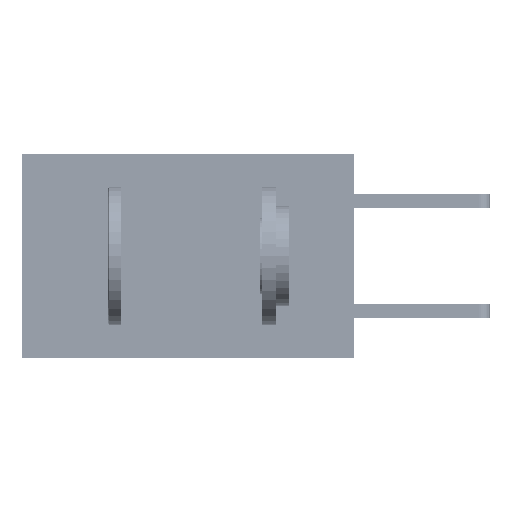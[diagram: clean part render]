
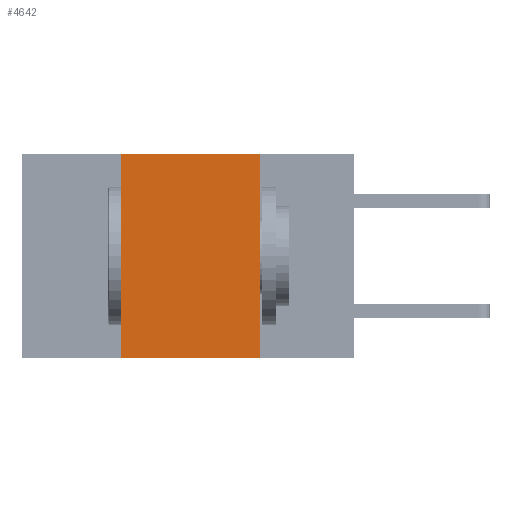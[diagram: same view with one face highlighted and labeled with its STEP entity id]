
A CAD part, left-side view. The second image highlights one B-rep face of the part: STEP entity #4642.
In plain terms, the highlighted planar face has unit normal (-1, 0, 0).
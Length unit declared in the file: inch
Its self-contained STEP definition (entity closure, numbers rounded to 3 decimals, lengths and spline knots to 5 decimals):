
#1347 = VERTEX_POINT ( 'NONE', #31128 ) ;
#1483 = CARTESIAN_POINT ( 'NONE',  ( 0., 0.17, 0. ) ) ;
#2092 = DIRECTION ( 'NONE',  ( 1., 0., 0. ) ) ;
#2954 = LINE ( 'NONE', #18787, #37682 ) ;
#4218 = DIRECTION ( 'NONE',  ( 0., -1., 0. ) ) ;
#4642 = ADVANCED_FACE ( 'NONE', ( #6497 ), #38147, .F. ) ;
#6009 = ORIENTED_EDGE ( 'NONE', *, *, #40248, .F. ) ;
#6497 = FACE_OUTER_BOUND ( 'NONE', #8638, .T. ) ;
#8426 = VERTEX_POINT ( 'NONE', #46338 ) ;
#8638 = EDGE_LOOP ( 'NONE', ( #23940, #8765, #6009, #19780 ) ) ;
#8765 = ORIENTED_EDGE ( 'NONE', *, *, #28833, .F. ) ;
#12913 = LINE ( 'NONE', #1483, #31798 ) ;
#18787 = CARTESIAN_POINT ( 'NONE',  ( 0., 0.6, 0. ) ) ;
#19563 = DIRECTION ( 'NONE',  ( 0., -1., 0. ) ) ;
#19780 = ORIENTED_EDGE ( 'NONE', *, *, #46282, .T. ) ;
#19797 = LINE ( 'NONE', #47793, #23349 ) ;
#20001 = CARTESIAN_POINT ( 'NONE',  ( 0., 0.42, 0. ) ) ;
#20131 = CARTESIAN_POINT ( 'NONE',  ( 0., 0.42, -0.37 ) ) ;
#23349 = VECTOR ( 'NONE', #4218, 39.37008 ) ;
#23940 = ORIENTED_EDGE ( 'NONE', *, *, #50758, .F. ) ;
#24908 = VERTEX_POINT ( 'NONE', #20001 ) ;
#26074 = CARTESIAN_POINT ( 'NONE',  ( 0., 0.42, 0. ) ) ;
#27103 = VERTEX_POINT ( 'NONE', #20131 ) ;
#28759 = DIRECTION ( 'NONE',  ( 0., 0., -1. ) ) ;
#28833 = EDGE_CURVE ( 'NONE', #24908, #1347, #2954, .T. ) ;
#30887 = CARTESIAN_POINT ( 'NONE',  ( 0., 0.6, 0. ) ) ;
#30989 = AXIS2_PLACEMENT_3D ( 'NONE', #30887, #2092, #46162 ) ;
#31128 = CARTESIAN_POINT ( 'NONE',  ( 0., 0.17, 0. ) ) ;
#31798 = VECTOR ( 'NONE', #28759, 39.37008 ) ;
#37682 = VECTOR ( 'NONE', #19563, 39.37008 ) ;
#37989 = DIRECTION ( 'NONE',  ( 0., 0., 1. ) ) ;
#38147 = PLANE ( 'NONE',  #30989 ) ;
#40248 = EDGE_CURVE ( 'NONE', #27103, #24908, #45764, .T. ) ;
#42134 = VECTOR ( 'NONE', #37989, 39.37008 ) ;
#45764 = LINE ( 'NONE', #26074, #42134 ) ;
#46162 = DIRECTION ( 'NONE',  ( 0., 0., -1. ) ) ;
#46282 = EDGE_CURVE ( 'NONE', #27103, #8426, #19797, .T. ) ;
#46338 = CARTESIAN_POINT ( 'NONE',  ( 0., 0.17, -0.37 ) ) ;
#47793 = CARTESIAN_POINT ( 'NONE',  ( 0., 0.6, -0.37 ) ) ;
#50758 = EDGE_CURVE ( 'NONE', #1347, #8426, #12913, .T. ) ;
